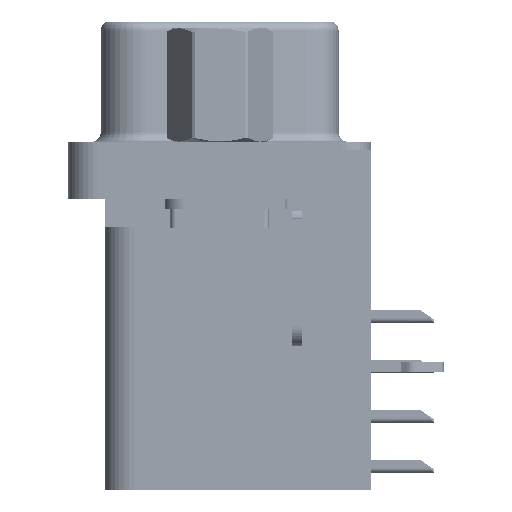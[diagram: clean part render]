
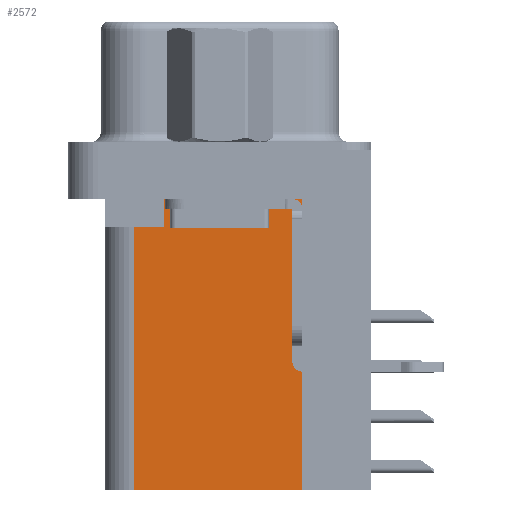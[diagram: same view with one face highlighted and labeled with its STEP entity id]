
A CAD part, left-side view. The second image highlights one B-rep face of the part: STEP entity #2572.
In plain terms, the highlighted planar face has unit normal (-1, 0, 0).
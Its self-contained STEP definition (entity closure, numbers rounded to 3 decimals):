
#1911 = EDGE_LOOP ( 'NONE', ( #32369, #33004, #7704, #33415, #11957, #38343 ) ) ;
#2572 = ADVANCED_FACE ( 'NONE', ( #37232 ), #4933, .F. ) ;
#3105 = CARTESIAN_POINT ( 'NONE',  ( 3.75, -4.2, -17.3 ) ) ;
#3929 = VERTEX_POINT ( 'NONE', #5729 ) ;
#4933 = PLANE ( 'NONE',  #26814 ) ;
#5542 = VECTOR ( 'NONE', #23847, 1000. ) ;
#5729 = CARTESIAN_POINT ( 'NONE',  ( 3.75, -4.2, -2.5 ) ) ;
#7000 = EDGE_CURVE ( 'NONE', #3929, #13240, #43485, .T. ) ;
#7494 = LINE ( 'NONE', #25890, #15994 ) ;
#7704 = ORIENTED_EDGE ( 'NONE', *, *, #32209, .T. ) ;
#7961 = DIRECTION ( 'NONE',  ( 0., 1., 0. ) ) ;
#8062 = DIRECTION ( 'NONE',  ( 0., 0., 1. ) ) ;
#9533 = EDGE_CURVE ( 'NONE', #28941, #19735, #22514, .T. ) ;
#11957 = ORIENTED_EDGE ( 'NONE', *, *, #14025, .F. ) ;
#12623 = VECTOR ( 'NONE', #24755, 1000. ) ;
#12878 = CARTESIAN_POINT ( 'NONE',  ( 3.75, -4.2, -2.5 ) ) ;
#13240 = VERTEX_POINT ( 'NONE', #41833 ) ;
#13482 = LINE ( 'NONE', #44528, #21850 ) ;
#14025 = EDGE_CURVE ( 'NONE', #25825, #28941, #40942, .T. ) ;
#14130 = CARTESIAN_POINT ( 'NONE',  ( 3.75, 2.85, -3.9 ) ) ;
#14476 = EDGE_CURVE ( 'NONE', #25825, #3929, #13482, .T. ) ;
#15219 = LINE ( 'NONE', #16661, #5542 ) ;
#15356 = CARTESIAN_POINT ( 'NONE',  ( 3.75, 4.35, -17.3 ) ) ;
#15994 = VECTOR ( 'NONE', #7961, 1000. ) ;
#16661 = CARTESIAN_POINT ( 'NONE',  ( 3.75, 2.85, -3.9 ) ) ;
#16742 = CARTESIAN_POINT ( 'NONE',  ( 3.75, -4.2, -17.3 ) ) ;
#19735 = VERTEX_POINT ( 'NONE', #43076 ) ;
#19921 = DIRECTION ( 'NONE',  ( 0., 0., 1. ) ) ;
#20919 = EDGE_CURVE ( 'NONE', #13240, #41647, #15219, .T. ) ;
#21279 = CARTESIAN_POINT ( 'NONE',  ( 3.75, -4.2, -17.3 ) ) ;
#21850 = VECTOR ( 'NONE', #19921, 1000. ) ;
#22514 = LINE ( 'NONE', #15356, #40227 ) ;
#23847 = DIRECTION ( 'NONE',  ( 0., 0., -1. ) ) ;
#24755 = DIRECTION ( 'NONE',  ( 0., 1., 0. ) ) ;
#25825 = VERTEX_POINT ( 'NONE', #16742 ) ;
#25890 = CARTESIAN_POINT ( 'NONE',  ( 3.75, 0., -3.9 ) ) ;
#26814 = AXIS2_PLACEMENT_3D ( 'NONE', #21279, #31213, #45950 ) ;
#28941 = VERTEX_POINT ( 'NONE', #41639 ) ;
#31213 = DIRECTION ( 'NONE',  ( 1., 0., 0. ) ) ;
#32209 = EDGE_CURVE ( 'NONE', #41647, #19735, #7494, .T. ) ;
#32369 = ORIENTED_EDGE ( 'NONE', *, *, #7000, .T. ) ;
#33004 = ORIENTED_EDGE ( 'NONE', *, *, #20919, .T. ) ;
#33415 = ORIENTED_EDGE ( 'NONE', *, *, #9533, .F. ) ;
#34161 = DIRECTION ( 'NONE',  ( 0., 1., 0. ) ) ;
#35166 = VECTOR ( 'NONE', #34161, 1000. ) ;
#37232 = FACE_OUTER_BOUND ( 'NONE', #1911, .T. ) ;
#38343 = ORIENTED_EDGE ( 'NONE', *, *, #14476, .T. ) ;
#40227 = VECTOR ( 'NONE', #8062, 1000. ) ;
#40942 = LINE ( 'NONE', #3105, #12623 ) ;
#41639 = CARTESIAN_POINT ( 'NONE',  ( 3.75, 4.35, -17.3 ) ) ;
#41647 = VERTEX_POINT ( 'NONE', #14130 ) ;
#41833 = CARTESIAN_POINT ( 'NONE',  ( 3.75, 2.85, -2.5 ) ) ;
#43076 = CARTESIAN_POINT ( 'NONE',  ( 3.75, 4.35, -3.9 ) ) ;
#43485 = LINE ( 'NONE', #12878, #35166 ) ;
#44528 = CARTESIAN_POINT ( 'NONE',  ( 3.75, -4.2, -17.3 ) ) ;
#45950 = DIRECTION ( 'NONE',  ( 0., 1., 0. ) ) ;
